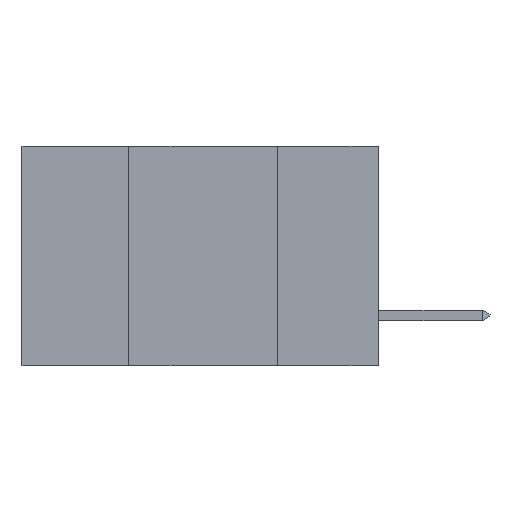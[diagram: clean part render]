
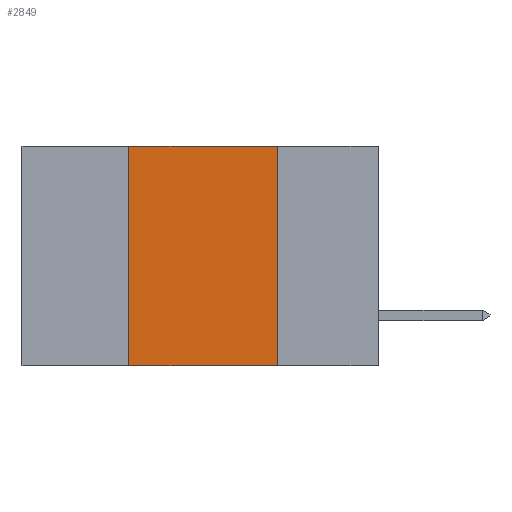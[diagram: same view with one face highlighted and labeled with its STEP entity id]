
A CAD part, left-side view. The second image highlights one B-rep face of the part: STEP entity #2849.
In plain terms, the highlighted planar face has unit normal (-1, 0, 0).
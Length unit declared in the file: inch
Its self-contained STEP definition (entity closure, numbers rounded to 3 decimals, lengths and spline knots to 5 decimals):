
#66 = DIRECTION ( 'NONE',  ( 0., 0., 1. ) ) ;
#221 = DIRECTION ( 'NONE',  ( 0., -1., 0. ) ) ;
#500 = CARTESIAN_POINT ( 'NONE',  ( 0., 0.17, 0. ) ) ;
#820 = CARTESIAN_POINT ( 'NONE',  ( 0., 0.6, 0. ) ) ;
#854 = LINE ( 'NONE', #9171, #7819 ) ;
#1034 = VERTEX_POINT ( 'NONE', #3475 ) ;
#1114 = PLANE ( 'NONE',  #3187 ) ;
#1154 = CARTESIAN_POINT ( 'NONE',  ( 0., 0.17, -0.37 ) ) ;
#1287 = VERTEX_POINT ( 'NONE', #3221 ) ;
#1293 = EDGE_CURVE ( 'NONE', #1034, #1287, #7676, .T. ) ;
#1454 = EDGE_LOOP ( 'NONE', ( #5082, #5385, #7584, #2562 ) ) ;
#1654 = VECTOR ( 'NONE', #6302, 39.37008 ) ;
#1799 = LINE ( 'NONE', #1154, #1654 ) ;
#2359 = LINE ( 'NONE', #820, #9668 ) ;
#2456 = DIRECTION ( 'NONE',  ( 0., -1., 0. ) ) ;
#2489 = CARTESIAN_POINT ( 'NONE',  ( 0., 0.42, -0.37 ) ) ;
#2562 = ORIENTED_EDGE ( 'NONE', *, *, #6505, .T. ) ;
#2649 = EDGE_CURVE ( 'NONE', #1287, #3703, #2359, .T. ) ;
#2849 = ADVANCED_FACE ( 'NONE', ( #3480 ), #1114, .F. ) ;
#3116 = EDGE_CURVE ( 'NONE', #3703, #7970, #1799, .T. ) ;
#3187 = AXIS2_PLACEMENT_3D ( 'NONE', #4821, #4133, #4088 ) ;
#3221 = CARTESIAN_POINT ( 'NONE',  ( 0., 0.42, 0. ) ) ;
#3475 = CARTESIAN_POINT ( 'NONE',  ( 0., 0.42, -0.37 ) ) ;
#3480 = FACE_OUTER_BOUND ( 'NONE', #1454, .T. ) ;
#3703 = VERTEX_POINT ( 'NONE', #500 ) ;
#4088 = DIRECTION ( 'NONE',  ( 0., 0., -1. ) ) ;
#4133 = DIRECTION ( 'NONE',  ( 1., 0., 0. ) ) ;
#4821 = CARTESIAN_POINT ( 'NONE',  ( 0., 0.6, 0. ) ) ;
#4953 = CARTESIAN_POINT ( 'NONE',  ( 0., 0.17, -0.37 ) ) ;
#5082 = ORIENTED_EDGE ( 'NONE', *, *, #3116, .F. ) ;
#5385 = ORIENTED_EDGE ( 'NONE', *, *, #2649, .F. ) ;
#6302 = DIRECTION ( 'NONE',  ( 0., 0., -1. ) ) ;
#6505 = EDGE_CURVE ( 'NONE', #1034, #7970, #854, .T. ) ;
#7325 = VECTOR ( 'NONE', #66, 39.37008 ) ;
#7584 = ORIENTED_EDGE ( 'NONE', *, *, #1293, .F. ) ;
#7676 = LINE ( 'NONE', #2489, #7325 ) ;
#7819 = VECTOR ( 'NONE', #221, 39.37008 ) ;
#7970 = VERTEX_POINT ( 'NONE', #4953 ) ;
#9171 = CARTESIAN_POINT ( 'NONE',  ( 0., 0.6, -0.37 ) ) ;
#9668 = VECTOR ( 'NONE', #2456, 39.37008 ) ;
